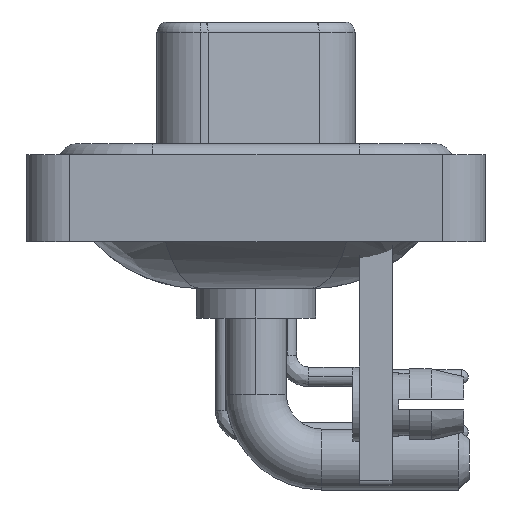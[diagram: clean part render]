
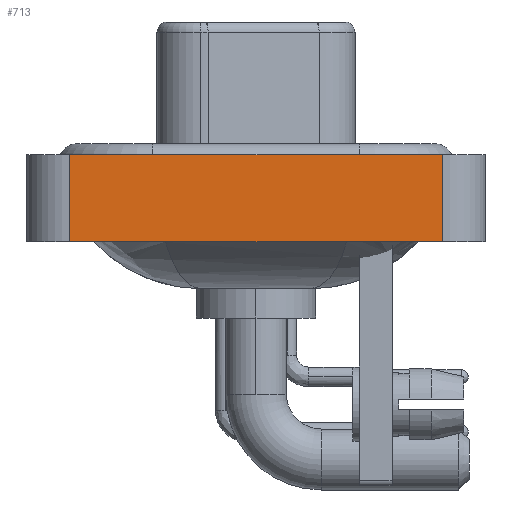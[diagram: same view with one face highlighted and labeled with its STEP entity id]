
A CAD part, left-side view. The second image highlights one B-rep face of the part: STEP entity #713.
In plain terms, the highlighted planar face has unit normal (-1, 0, 0).
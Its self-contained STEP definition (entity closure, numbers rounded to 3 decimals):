
#571 = VERTEX_POINT ( 'NONE', #2741 ) ;
#713 = ADVANCED_FACE ( 'NONE', ( #17276 ), #18937, .T. ) ;
#2207 = VERTEX_POINT ( 'NONE', #22686 ) ;
#2741 = CARTESIAN_POINT ( 'NONE',  ( -7.35, 8.55, 0.4 ) ) ;
#2914 = EDGE_CURVE ( 'NONE', #2207, #571, #16770, .T. ) ;
#3337 = VERTEX_POINT ( 'NONE', #21083 ) ;
#5006 = DIRECTION ( 'NONE',  ( 0., -1., 0. ) ) ;
#6852 = LINE ( 'NONE', #11493, #15280 ) ;
#9355 = LINE ( 'NONE', #18663, #10388 ) ;
#9745 = ORIENTED_EDGE ( 'NONE', *, *, #11950, .F. ) ;
#9956 = VERTEX_POINT ( 'NONE', #23701 ) ;
#10388 = VECTOR ( 'NONE', #5006, 1000. ) ;
#11493 = CARTESIAN_POINT ( 'NONE',  ( -7.35, -8.55, -3.6 ) ) ;
#11950 = EDGE_CURVE ( 'NONE', #571, #9956, #26026, .T. ) ;
#12048 = DIRECTION ( 'NONE',  ( 0., -1., 0. ) ) ;
#12329 = DIRECTION ( 'NONE',  ( -1., 0., 0. ) ) ;
#13084 = VECTOR ( 'NONE', #28352, 1000. ) ;
#14730 = CARTESIAN_POINT ( 'NONE',  ( -7.35, -8.55, -3.6 ) ) ;
#15280 = VECTOR ( 'NONE', #20645, 1000. ) ;
#15903 = EDGE_LOOP ( 'NONE', ( #16185, #9745, #19350, #20577 ) ) ;
#16185 = ORIENTED_EDGE ( 'NONE', *, *, #28482, .T. ) ;
#16770 = LINE ( 'NONE', #25942, #13084 ) ;
#17276 = FACE_OUTER_BOUND ( 'NONE', #15903, .T. ) ;
#18663 = CARTESIAN_POINT ( 'NONE',  ( -7.35, -8.55, -3.6 ) ) ;
#18937 = PLANE ( 'NONE',  #19048 ) ;
#19048 = AXIS2_PLACEMENT_3D ( 'NONE', #14730, #12329, #26161 ) ;
#19350 = ORIENTED_EDGE ( 'NONE', *, *, #2914, .F. ) ;
#20577 = ORIENTED_EDGE ( 'NONE', *, *, #24904, .T. ) ;
#20645 = DIRECTION ( 'NONE',  ( 0., 0., 1. ) ) ;
#21083 = CARTESIAN_POINT ( 'NONE',  ( -7.35, -8.55, -3.6 ) ) ;
#22686 = CARTESIAN_POINT ( 'NONE',  ( -7.35, 8.55, -3.6 ) ) ;
#23701 = CARTESIAN_POINT ( 'NONE',  ( -7.35, -8.55, 0.4 ) ) ;
#24904 = EDGE_CURVE ( 'NONE', #2207, #3337, #9355, .T. ) ;
#25870 = CARTESIAN_POINT ( 'NONE',  ( -7.35, -8.55, 0.4 ) ) ;
#25942 = CARTESIAN_POINT ( 'NONE',  ( -7.35, 8.55, -3.6 ) ) ;
#26006 = VECTOR ( 'NONE', #12048, 1000. ) ;
#26026 = LINE ( 'NONE', #25870, #26006 ) ;
#26161 = DIRECTION ( 'NONE',  ( 0., 0., 1. ) ) ;
#28352 = DIRECTION ( 'NONE',  ( 0., 0., 1. ) ) ;
#28482 = EDGE_CURVE ( 'NONE', #3337, #9956, #6852, .T. ) ;
